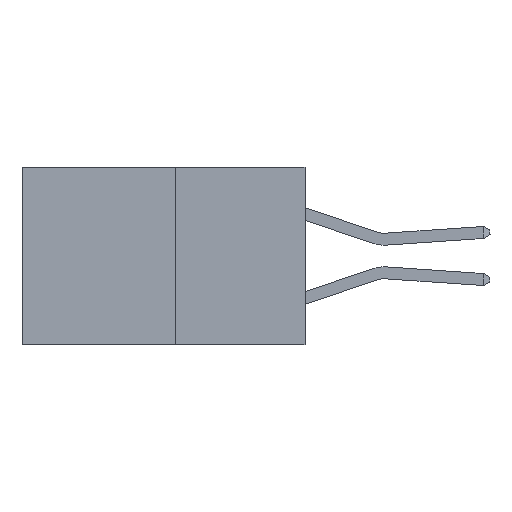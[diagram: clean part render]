
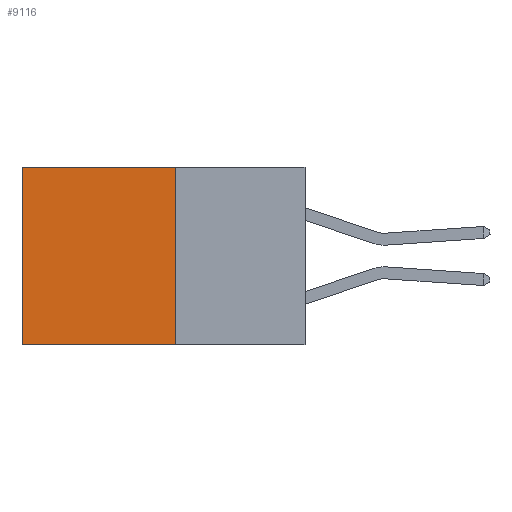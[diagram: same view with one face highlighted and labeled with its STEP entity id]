
A CAD part, left-side view. The second image highlights one B-rep face of the part: STEP entity #9116.
In plain terms, the highlighted planar face has unit normal (-1, 0, 0).
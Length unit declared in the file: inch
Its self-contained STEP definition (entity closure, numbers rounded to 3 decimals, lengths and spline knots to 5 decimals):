
#655 = PLANE ( 'NONE',  #24128 ) ;
#678 = LINE ( 'NONE', #3804, #11351 ) ;
#1612 = FACE_OUTER_BOUND ( 'NONE', #26787, .T. ) ;
#2928 = EDGE_CURVE ( 'NONE', #11589, #6688, #25287, .T. ) ;
#3804 = CARTESIAN_POINT ( 'NONE',  ( 0.277, 0.27, -0.37 ) ) ;
#3992 = CARTESIAN_POINT ( 'NONE',  ( 0.277, 0.59, -0.37 ) ) ;
#5129 = CARTESIAN_POINT ( 'NONE',  ( 0.277, 0.27, -0.37 ) ) ;
#5983 = CARTESIAN_POINT ( 'NONE',  ( 0.277, 0.59, 0. ) ) ;
#6223 = VERTEX_POINT ( 'NONE', #12538 ) ;
#6688 = VERTEX_POINT ( 'NONE', #5983 ) ;
#7263 = VECTOR ( 'NONE', #22849, 39.37008 ) ;
#7437 = VECTOR ( 'NONE', #19015, 39.37008 ) ;
#9116 = ADVANCED_FACE ( 'NONE', ( #1612 ), #655, .F. ) ;
#9374 = DIRECTION ( 'NONE',  ( 1., 0., 0. ) ) ;
#11201 = EDGE_CURVE ( 'NONE', #6223, #21659, #678, .T. ) ;
#11351 = VECTOR ( 'NONE', #16379, 39.37008 ) ;
#11589 = VERTEX_POINT ( 'NONE', #19705 ) ;
#12538 = CARTESIAN_POINT ( 'NONE',  ( 0.277, 0.27, -0.37 ) ) ;
#12898 = LINE ( 'NONE', #21255, #23313 ) ;
#15543 = CARTESIAN_POINT ( 'NONE',  ( 0.277, 0.59, -0.37 ) ) ;
#16379 = DIRECTION ( 'NONE',  ( 0., 1., 0. ) ) ;
#19015 = DIRECTION ( 'NONE',  ( 0., 1., 0. ) ) ;
#19248 = CARTESIAN_POINT ( 'NONE',  ( 0.277, 0.27, 0. ) ) ;
#19705 = CARTESIAN_POINT ( 'NONE',  ( 0.277, 0.27, 0. ) ) ;
#20386 = ORIENTED_EDGE ( 'NONE', *, *, #20732, .T. ) ;
#20732 = EDGE_CURVE ( 'NONE', #6688, #21659, #23852, .T. ) ;
#21255 = CARTESIAN_POINT ( 'NONE',  ( 0.277, 0.27, -0.37 ) ) ;
#21659 = VERTEX_POINT ( 'NONE', #15543 ) ;
#22849 = DIRECTION ( 'NONE',  ( 0., 0., -1. ) ) ;
#23313 = VECTOR ( 'NONE', #23354, 39.37008 ) ;
#23354 = DIRECTION ( 'NONE',  ( 0., 0., -1. ) ) ;
#23852 = LINE ( 'NONE', #3992, #7263 ) ;
#23913 = DIRECTION ( 'NONE',  ( 0., 0., -1. ) ) ;
#24128 = AXIS2_PLACEMENT_3D ( 'NONE', #5129, #9374, #23913 ) ;
#24658 = ORIENTED_EDGE ( 'NONE', *, *, #11201, .F. ) ;
#25287 = LINE ( 'NONE', #19248, #7437 ) ;
#26276 = EDGE_CURVE ( 'NONE', #11589, #6223, #12898, .T. ) ;
#26713 = ORIENTED_EDGE ( 'NONE', *, *, #26276, .F. ) ;
#26787 = EDGE_LOOP ( 'NONE', ( #20386, #24658, #26713, #26810 ) ) ;
#26810 = ORIENTED_EDGE ( 'NONE', *, *, #2928, .T. ) ;
